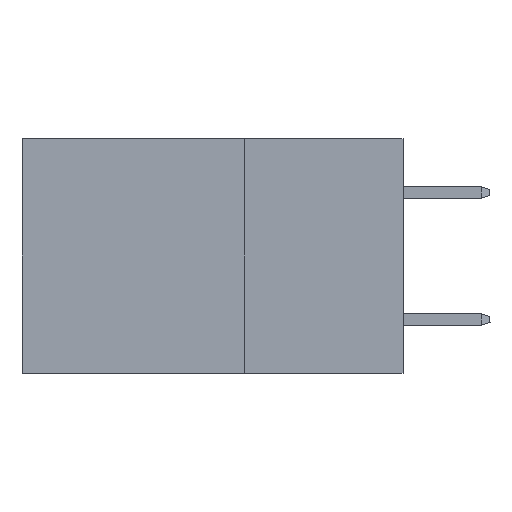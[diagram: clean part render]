
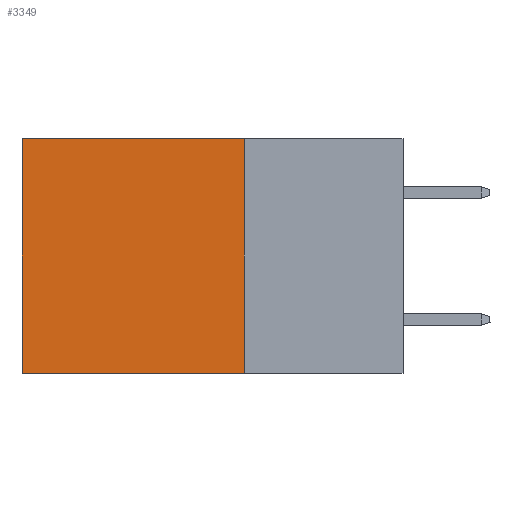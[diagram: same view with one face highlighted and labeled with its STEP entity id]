
A CAD part, left-side view. The second image highlights one B-rep face of the part: STEP entity #3349.
In plain terms, the highlighted planar face has unit normal (-1, 0, 0).
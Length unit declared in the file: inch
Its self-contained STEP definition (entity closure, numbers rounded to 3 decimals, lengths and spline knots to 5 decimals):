
#400 = CARTESIAN_POINT ( 'NONE',  ( 0.2875, 0.25, 0. ) ) ;
#488 = CARTESIAN_POINT ( 'NONE',  ( 0.2875, 0.25, 0. ) ) ;
#1219 = VERTEX_POINT ( 'NONE', #24311 ) ;
#1553 = EDGE_CURVE ( 'NONE', #24262, #23525, #19235, .T. ) ;
#2621 = LINE ( 'NONE', #22371, #24406 ) ;
#2723 = DIRECTION ( 'NONE',  ( 1., 0., 0. ) ) ;
#3124 = LINE ( 'NONE', #25475, #11327 ) ;
#3260 = VERTEX_POINT ( 'NONE', #13996 ) ;
#3349 = ADVANCED_FACE ( 'NONE', ( #13849 ), #24789, .F. ) ;
#4749 = DIRECTION ( 'NONE',  ( 0., 1., 0. ) ) ;
#6382 = EDGE_CURVE ( 'NONE', #23525, #3260, #3124, .T. ) ;
#6600 = LINE ( 'NONE', #488, #21413 ) ;
#6761 = EDGE_CURVE ( 'NONE', #24262, #1219, #6600, .T. ) ;
#9494 = DIRECTION ( 'NONE',  ( 0., 0., -1. ) ) ;
#10558 = EDGE_CURVE ( 'NONE', #1219, #3260, #2621, .T. ) ;
#11327 = VECTOR ( 'NONE', #11928, 39.37008 ) ;
#11928 = DIRECTION ( 'NONE',  ( 0., 0., -1. ) ) ;
#12827 = ORIENTED_EDGE ( 'NONE', *, *, #1553, .T. ) ;
#13770 = VECTOR ( 'NONE', #4749, 39.37008 ) ;
#13849 = FACE_OUTER_BOUND ( 'NONE', #20697, .T. ) ;
#13996 = CARTESIAN_POINT ( 'NONE',  ( 0.2875, 0.6, -0.37 ) ) ;
#14641 = ORIENTED_EDGE ( 'NONE', *, *, #10558, .F. ) ;
#15925 = DIRECTION ( 'NONE',  ( 0., 1., 0. ) ) ;
#16632 = AXIS2_PLACEMENT_3D ( 'NONE', #400, #2723, #9494 ) ;
#19235 = LINE ( 'NONE', #28004, #13770 ) ;
#20697 = EDGE_LOOP ( 'NONE', ( #21618, #14641, #25206, #12827 ) ) ;
#21413 = VECTOR ( 'NONE', #26605, 39.37008 ) ;
#21618 = ORIENTED_EDGE ( 'NONE', *, *, #6382, .T. ) ;
#22371 = CARTESIAN_POINT ( 'NONE',  ( 0.2875, 0.25, -0.37 ) ) ;
#23474 = CARTESIAN_POINT ( 'NONE',  ( 0.2875, 0.6, 0. ) ) ;
#23525 = VERTEX_POINT ( 'NONE', #23474 ) ;
#24262 = VERTEX_POINT ( 'NONE', #25126 ) ;
#24311 = CARTESIAN_POINT ( 'NONE',  ( 0.2875, 0.25, -0.37 ) ) ;
#24406 = VECTOR ( 'NONE', #15925, 39.37008 ) ;
#24789 = PLANE ( 'NONE',  #16632 ) ;
#25126 = CARTESIAN_POINT ( 'NONE',  ( 0.2875, 0.25, 0. ) ) ;
#25206 = ORIENTED_EDGE ( 'NONE', *, *, #6761, .F. ) ;
#25475 = CARTESIAN_POINT ( 'NONE',  ( 0.2875, 0.6, 0. ) ) ;
#26605 = DIRECTION ( 'NONE',  ( 0., 0., -1. ) ) ;
#28004 = CARTESIAN_POINT ( 'NONE',  ( 0.2875, 0.25, 0. ) ) ;
